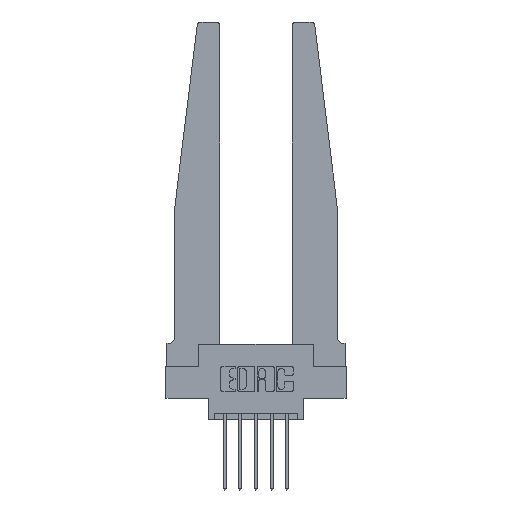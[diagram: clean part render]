
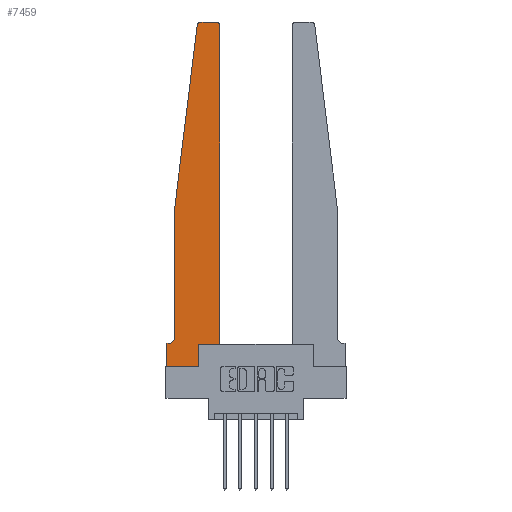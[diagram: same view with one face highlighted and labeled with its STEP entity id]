
A CAD part, top view. The second image highlights one B-rep face of the part: STEP entity #7459.
In plain terms, the highlighted planar face has unit normal (0, 0, 1).
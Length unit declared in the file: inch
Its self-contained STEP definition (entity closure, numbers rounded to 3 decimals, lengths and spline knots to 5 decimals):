
#59 = CARTESIAN_POINT ( 'NONE',  ( 0.065, 1.25, 0.37 ) ) ;
#233 = VERTEX_POINT ( 'NONE', #7249 ) ;
#340 = CARTESIAN_POINT ( 'NONE',  ( 0.015, 0.1875, 0.37 ) ) ;
#471 = EDGE_CURVE ( 'NONE', #5923, #3634, #3984, .T. ) ;
#688 = ORIENTED_EDGE ( 'NONE', *, *, #2064, .T. ) ;
#692 = CARTESIAN_POINT ( 'NONE',  ( 0.27653, 2.75, 0.37 ) ) ;
#722 = ORIENTED_EDGE ( 'NONE', *, *, #3627, .T. ) ;
#745 = DIRECTION ( 'NONE',  ( 0., 0., 1. ) ) ;
#766 = AXIS2_PLACEMENT_3D ( 'NONE', #9838, #1379, #4451 ) ;
#789 = CARTESIAN_POINT ( 'NONE',  ( 0., 0., 0.37 ) ) ;
#822 = ORIENTED_EDGE ( 'NONE', *, *, #471, .T. ) ;
#1029 = DIRECTION ( 'NONE',  ( 1., 0., 0. ) ) ;
#1055 = VERTEX_POINT ( 'NONE', #12806 ) ;
#1379 = DIRECTION ( 'NONE',  ( 0., 0., 1. ) ) ;
#1839 = VECTOR ( 'NONE', #12805, 39.37008 ) ;
#1883 = AXIS2_PLACEMENT_3D ( 'NONE', #11465, #10449, #1029 ) ;
#1915 = DIRECTION ( 'NONE',  ( 1., 0., 0. ) ) ;
#1957 = LINE ( 'NONE', #789, #4825 ) ;
#2064 = EDGE_CURVE ( 'NONE', #3634, #10814, #7502, .T. ) ;
#2285 = DIRECTION ( 'NONE',  ( 0., -1., 0. ) ) ;
#2613 = VERTEX_POINT ( 'NONE', #692 ) ;
#2738 = EDGE_LOOP ( 'NONE', ( #8477, #7994, #7522, #12056, #6442, #822, #688, #11734, #4629, #722, #9825, #10015 ) ) ;
#2944 = CARTESIAN_POINT ( 'NONE',  ( 0.425, 0.18, 0.37 ) ) ;
#3077 = CARTESIAN_POINT ( 'NONE',  ( 0., 0.1875, 0.37 ) ) ;
#3342 = EDGE_CURVE ( 'NONE', #8361, #233, #7412, .T. ) ;
#3515 = DIRECTION ( 'NONE',  ( -1., 0., 0. ) ) ;
#3627 = EDGE_CURVE ( 'NONE', #13353, #1055, #9195, .T. ) ;
#3634 = VERTEX_POINT ( 'NONE', #3077 ) ;
#3667 = DIRECTION ( 'NONE',  ( 0., 1., 0. ) ) ;
#3984 = LINE ( 'NONE', #6192, #13393 ) ;
#3997 = EDGE_CURVE ( 'NONE', #10814, #13352, #1957, .T. ) ;
#4004 = DIRECTION ( 'NONE',  ( 1., 0., 0. ) ) ;
#4366 = LINE ( 'NONE', #5278, #7356 ) ;
#4451 = DIRECTION ( 'NONE',  ( 1., 0., 0. ) ) ;
#4629 = ORIENTED_EDGE ( 'NONE', *, *, #8920, .T. ) ;
#4825 = VECTOR ( 'NONE', #4967, 39.37008 ) ;
#4967 = DIRECTION ( 'NONE',  ( 1., 0., 0. ) ) ;
#5132 = CIRCLE ( 'NONE', #766, 0.03 ) ;
#5278 = CARTESIAN_POINT ( 'NONE',  ( 0.425, 0.18, 0.37 ) ) ;
#5440 = EDGE_CURVE ( 'NONE', #9642, #5923, #6912, .T. ) ;
#5742 = LINE ( 'NONE', #6979, #10856 ) ;
#5923 = VERTEX_POINT ( 'NONE', #340 ) ;
#6158 = CARTESIAN_POINT ( 'NONE',  ( 0., 0.1875, 0.37 ) ) ;
#6192 = CARTESIAN_POINT ( 'NONE',  ( 0.065, 0.1875, 0.37 ) ) ;
#6343 = LINE ( 'NONE', #8478, #1839 ) ;
#6432 = VECTOR ( 'NONE', #2285, 39.37008 ) ;
#6442 = ORIENTED_EDGE ( 'NONE', *, *, #5440, .T. ) ;
#6546 = CARTESIAN_POINT ( 'NONE',  ( 0., 0., 0.37 ) ) ;
#6912 = CIRCLE ( 'NONE', #8899, 0.05 ) ;
#6979 = CARTESIAN_POINT ( 'NONE',  ( 0.2605, 0.18, 0.37 ) ) ;
#7249 = CARTESIAN_POINT ( 'NONE',  ( 0.065, 1.25, 0.37 ) ) ;
#7302 = LINE ( 'NONE', #11501, #13542 ) ;
#7356 = VECTOR ( 'NONE', #12641, 39.37008 ) ;
#7412 = LINE ( 'NONE', #59, #11230 ) ;
#7459 = ADVANCED_FACE ( 'NONE', ( #9337 ), #13538, .T. ) ;
#7502 = LINE ( 'NONE', #11696, #6432 ) ;
#7522 = ORIENTED_EDGE ( 'NONE', *, *, #3342, .T. ) ;
#7796 = CIRCLE ( 'NONE', #1883, 0.03 ) ;
#7986 = EDGE_CURVE ( 'NONE', #233, #9642, #6343, .T. ) ;
#7994 = ORIENTED_EDGE ( 'NONE', *, *, #11702, .T. ) ;
#8358 = CARTESIAN_POINT ( 'NONE',  ( 0.2605, 0.18, 0.37 ) ) ;
#8361 = VERTEX_POINT ( 'NONE', #10399 ) ;
#8404 = AXIS2_PLACEMENT_3D ( 'NONE', #6158, #745, #1915 ) ;
#8477 = ORIENTED_EDGE ( 'NONE', *, *, #10764, .T. ) ;
#8478 = CARTESIAN_POINT ( 'NONE',  ( 0.065, 1.25, 0.37 ) ) ;
#8524 = EDGE_CURVE ( 'NONE', #10845, #9708, #5132, .T. ) ;
#8899 = AXIS2_PLACEMENT_3D ( 'NONE', #10743, #12939, #3515 ) ;
#8920 = EDGE_CURVE ( 'NONE', #13352, #13353, #5742, .T. ) ;
#9195 = LINE ( 'NONE', #2944, #9858 ) ;
#9337 = FACE_OUTER_BOUND ( 'NONE', #2738, .T. ) ;
#9642 = VERTEX_POINT ( 'NONE', #12793 ) ;
#9708 = VERTEX_POINT ( 'NONE', #10664 ) ;
#9825 = ORIENTED_EDGE ( 'NONE', *, *, #11640, .T. ) ;
#9838 = CARTESIAN_POINT ( 'NONE',  ( 0.395, 2.72, 0.37 ) ) ;
#9858 = VECTOR ( 'NONE', #4004, 39.37008 ) ;
#10015 = ORIENTED_EDGE ( 'NONE', *, *, #8524, .T. ) ;
#10399 = CARTESIAN_POINT ( 'NONE',  ( 0.24675, 2.72367, 0.37 ) ) ;
#10449 = DIRECTION ( 'NONE',  ( 0., 0., 1. ) ) ;
#10664 = CARTESIAN_POINT ( 'NONE',  ( 0.395, 2.75, 0.37 ) ) ;
#10743 = CARTESIAN_POINT ( 'NONE',  ( 0.015, 0.2375, 0.37 ) ) ;
#10764 = EDGE_CURVE ( 'NONE', #9708, #2613, #7302, .T. ) ;
#10769 = DIRECTION ( 'NONE',  ( -0.122, -0.992, 0. ) ) ;
#10814 = VERTEX_POINT ( 'NONE', #6546 ) ;
#10845 = VERTEX_POINT ( 'NONE', #12874 ) ;
#10856 = VECTOR ( 'NONE', #3667, 39.37008 ) ;
#11230 = VECTOR ( 'NONE', #10769, 39.37008 ) ;
#11465 = CARTESIAN_POINT ( 'NONE',  ( 0.27653, 2.72, 0.37 ) ) ;
#11501 = CARTESIAN_POINT ( 'NONE',  ( 0.25, 2.75, 0.37 ) ) ;
#11640 = EDGE_CURVE ( 'NONE', #1055, #10845, #4366, .T. ) ;
#11696 = CARTESIAN_POINT ( 'NONE',  ( 0., 0., 0.37 ) ) ;
#11702 = EDGE_CURVE ( 'NONE', #2613, #8361, #7796, .T. ) ;
#11724 = CARTESIAN_POINT ( 'NONE',  ( 0.2605, 0., 0.37 ) ) ;
#11734 = ORIENTED_EDGE ( 'NONE', *, *, #3997, .T. ) ;
#12056 = ORIENTED_EDGE ( 'NONE', *, *, #7986, .T. ) ;
#12410 = DIRECTION ( 'NONE',  ( -1., 0., 0. ) ) ;
#12595 = DIRECTION ( 'NONE',  ( -1., 0., 0. ) ) ;
#12641 = DIRECTION ( 'NONE',  ( 0., 1., 0. ) ) ;
#12793 = CARTESIAN_POINT ( 'NONE',  ( 0.065, 0.2375, 0.37 ) ) ;
#12805 = DIRECTION ( 'NONE',  ( 0., -1., 0. ) ) ;
#12806 = CARTESIAN_POINT ( 'NONE',  ( 0.425, 0.18, 0.37 ) ) ;
#12874 = CARTESIAN_POINT ( 'NONE',  ( 0.425, 2.72, 0.37 ) ) ;
#12939 = DIRECTION ( 'NONE',  ( 0., 0., -1. ) ) ;
#13352 = VERTEX_POINT ( 'NONE', #11724 ) ;
#13353 = VERTEX_POINT ( 'NONE', #8358 ) ;
#13393 = VECTOR ( 'NONE', #12595, 39.37008 ) ;
#13538 = PLANE ( 'NONE',  #8404 ) ;
#13542 = VECTOR ( 'NONE', #12410, 39.37008 ) ;
